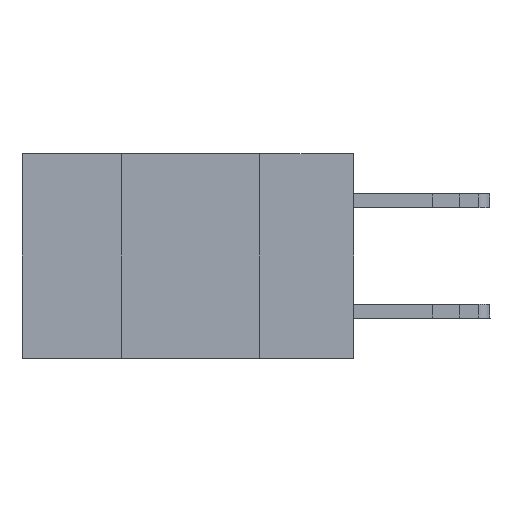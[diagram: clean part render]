
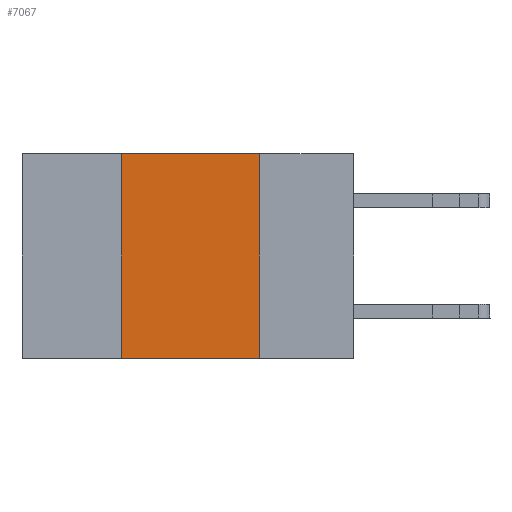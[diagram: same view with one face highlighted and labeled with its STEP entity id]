
A CAD part, left-side view. The second image highlights one B-rep face of the part: STEP entity #7067.
In plain terms, the highlighted planar face has unit normal (-1, 0, 0).
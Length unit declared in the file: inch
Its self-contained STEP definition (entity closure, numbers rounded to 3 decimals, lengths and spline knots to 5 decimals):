
#300 = ORIENTED_EDGE ( 'NONE', *, *, #14689, .F. ) ;
#544 = PLANE ( 'NONE',  #14312 ) ;
#806 = ORIENTED_EDGE ( 'NONE', *, *, #5053, .F. ) ;
#1142 = ORIENTED_EDGE ( 'NONE', *, *, #6259, .F. ) ;
#1441 = EDGE_CURVE ( 'NONE', #2765, #22724, #4940, .T. ) ;
#1476 = ORIENTED_EDGE ( 'NONE', *, *, #1441, .T. ) ;
#2496 = DIRECTION ( 'NONE',  ( 1., 0., 0. ) ) ;
#2765 = VERTEX_POINT ( 'NONE', #16273 ) ;
#2901 = VECTOR ( 'NONE', #6890, 39.37008 ) ;
#4785 = DIRECTION ( 'NONE',  ( 0., 0., -1. ) ) ;
#4940 = LINE ( 'NONE', #6287, #23100 ) ;
#5053 = EDGE_CURVE ( 'NONE', #14951, #5253, #22808, .T. ) ;
#5253 = VERTEX_POINT ( 'NONE', #7836 ) ;
#6259 = EDGE_CURVE ( 'NONE', #2765, #14951, #10259, .T. ) ;
#6287 = CARTESIAN_POINT ( 'NONE',  ( 0., 0.6, -0.37 ) ) ;
#6689 = CARTESIAN_POINT ( 'NONE',  ( 0., 0.17, -0.37 ) ) ;
#6890 = DIRECTION ( 'NONE',  ( 0., -1., 0. ) ) ;
#7067 = ADVANCED_FACE ( 'NONE', ( #21036 ), #544, .F. ) ;
#7836 = CARTESIAN_POINT ( 'NONE',  ( 0., 0.17, 0. ) ) ;
#8976 = DIRECTION ( 'NONE',  ( 0., 0., 1. ) ) ;
#10259 = LINE ( 'NONE', #19862, #20490 ) ;
#13683 = LINE ( 'NONE', #15572, #18527 ) ;
#14312 = AXIS2_PLACEMENT_3D ( 'NONE', #20616, #2496, #15152 ) ;
#14689 = EDGE_CURVE ( 'NONE', #5253, #22724, #13683, .T. ) ;
#14951 = VERTEX_POINT ( 'NONE', #21766 ) ;
#15152 = DIRECTION ( 'NONE',  ( 0., 0., -1. ) ) ;
#15572 = CARTESIAN_POINT ( 'NONE',  ( 0., 0.17, 0. ) ) ;
#16273 = CARTESIAN_POINT ( 'NONE',  ( 0., 0.42, -0.37 ) ) ;
#17986 = EDGE_LOOP ( 'NONE', ( #300, #806, #1142, #1476 ) ) ;
#18527 = VECTOR ( 'NONE', #4785, 39.37008 ) ;
#19578 = CARTESIAN_POINT ( 'NONE',  ( 0., 0.6, 0. ) ) ;
#19862 = CARTESIAN_POINT ( 'NONE',  ( 0., 0.42, 0. ) ) ;
#20490 = VECTOR ( 'NONE', #8976, 39.37008 ) ;
#20616 = CARTESIAN_POINT ( 'NONE',  ( 0., 0.6, 0. ) ) ;
#20967 = DIRECTION ( 'NONE',  ( 0., -1., 0. ) ) ;
#21036 = FACE_OUTER_BOUND ( 'NONE', #17986, .T. ) ;
#21766 = CARTESIAN_POINT ( 'NONE',  ( 0., 0.42, 0. ) ) ;
#22724 = VERTEX_POINT ( 'NONE', #6689 ) ;
#22808 = LINE ( 'NONE', #19578, #2901 ) ;
#23100 = VECTOR ( 'NONE', #20967, 39.37008 ) ;
